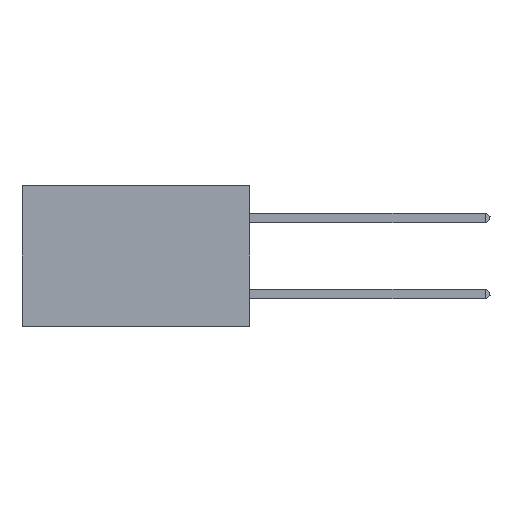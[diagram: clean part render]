
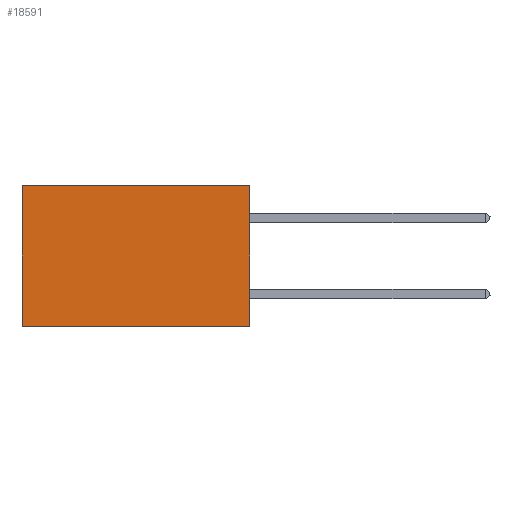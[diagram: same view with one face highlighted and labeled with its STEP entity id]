
A CAD part, left-side view. The second image highlights one B-rep face of the part: STEP entity #18591.
In plain terms, the highlighted planar face has unit normal (-1, 0, 0).
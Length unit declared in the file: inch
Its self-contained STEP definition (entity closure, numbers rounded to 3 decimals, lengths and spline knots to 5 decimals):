
#26 = LINE ( 'NONE', #28043, #22105 ) ;
#3866 = CARTESIAN_POINT ( 'NONE',  ( 0.2875, 0., 0. ) ) ;
#4439 = VERTEX_POINT ( 'NONE', #5180 ) ;
#5180 = CARTESIAN_POINT ( 'NONE',  ( 0.2875, 0., -0.37 ) ) ;
#7383 = VECTOR ( 'NONE', #12118, 39.37008 ) ;
#8693 = AXIS2_PLACEMENT_3D ( 'NONE', #32381, #12243, #9229 ) ;
#8842 = VECTOR ( 'NONE', #35829, 39.37008 ) ;
#9166 = CARTESIAN_POINT ( 'NONE',  ( 0.2875, 0.6, -0.37 ) ) ;
#9229 = DIRECTION ( 'NONE',  ( 0., 0., -1. ) ) ;
#12118 = DIRECTION ( 'NONE',  ( 0., 1., 0. ) ) ;
#12243 = DIRECTION ( 'NONE',  ( 1., 0., 0. ) ) ;
#12355 = EDGE_CURVE ( 'NONE', #13667, #19753, #13219, .T. ) ;
#13219 = LINE ( 'NONE', #28425, #37052 ) ;
#13443 = DIRECTION ( 'NONE',  ( 0., 0., -1. ) ) ;
#13667 = VERTEX_POINT ( 'NONE', #14210 ) ;
#13751 = VERTEX_POINT ( 'NONE', #9166 ) ;
#14102 = DIRECTION ( 'NONE',  ( 0., 1., 0. ) ) ;
#14210 = CARTESIAN_POINT ( 'NONE',  ( 0.2875, 0., 0. ) ) ;
#14868 = ORIENTED_EDGE ( 'NONE', *, *, #12355, .T. ) ;
#15047 = LINE ( 'NONE', #18179, #7383 ) ;
#18179 = CARTESIAN_POINT ( 'NONE',  ( 0.2875, 0., -0.37 ) ) ;
#18591 = ADVANCED_FACE ( 'NONE', ( #35493 ), #26105, .F. ) ;
#19593 = EDGE_CURVE ( 'NONE', #13667, #4439, #26881, .T. ) ;
#19753 = VERTEX_POINT ( 'NONE', #30803 ) ;
#22105 = VECTOR ( 'NONE', #13443, 39.37008 ) ;
#26105 = PLANE ( 'NONE',  #8693 ) ;
#26831 = EDGE_LOOP ( 'NONE', ( #32998, #26931, #27127, #14868 ) ) ;
#26881 = LINE ( 'NONE', #3866, #8842 ) ;
#26931 = ORIENTED_EDGE ( 'NONE', *, *, #32223, .F. ) ;
#27127 = ORIENTED_EDGE ( 'NONE', *, *, #19593, .F. ) ;
#28043 = CARTESIAN_POINT ( 'NONE',  ( 0.2875, 0.6, 0. ) ) ;
#28425 = CARTESIAN_POINT ( 'NONE',  ( 0.2875, 0., 0. ) ) ;
#30803 = CARTESIAN_POINT ( 'NONE',  ( 0.2875, 0.6, 0. ) ) ;
#32223 = EDGE_CURVE ( 'NONE', #4439, #13751, #15047, .T. ) ;
#32381 = CARTESIAN_POINT ( 'NONE',  ( 0.2875, 0., 0. ) ) ;
#32998 = ORIENTED_EDGE ( 'NONE', *, *, #35864, .T. ) ;
#35493 = FACE_OUTER_BOUND ( 'NONE', #26831, .T. ) ;
#35829 = DIRECTION ( 'NONE',  ( 0., 0., -1. ) ) ;
#35864 = EDGE_CURVE ( 'NONE', #19753, #13751, #26, .T. ) ;
#37052 = VECTOR ( 'NONE', #14102, 39.37008 ) ;
